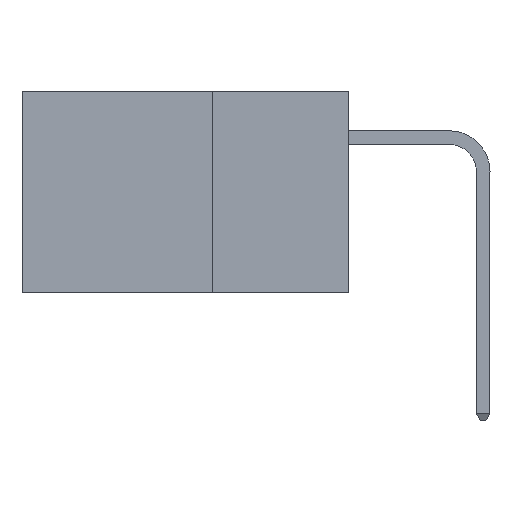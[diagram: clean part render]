
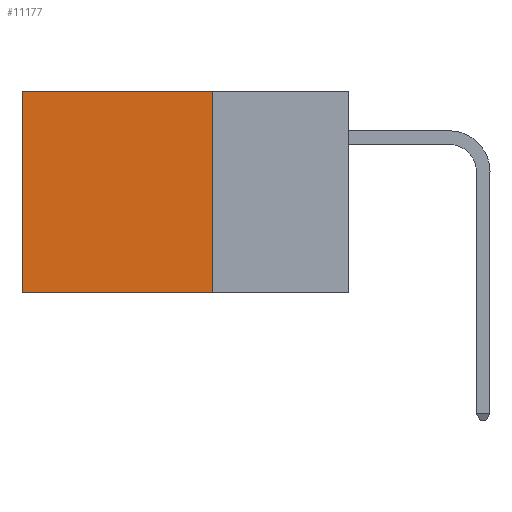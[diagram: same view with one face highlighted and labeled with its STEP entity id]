
A CAD part, left-side view. The second image highlights one B-rep face of the part: STEP entity #11177.
In plain terms, the highlighted planar face has unit normal (-1, 0, 0).
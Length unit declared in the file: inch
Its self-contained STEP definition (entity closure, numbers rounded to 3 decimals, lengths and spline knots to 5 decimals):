
#1679 = VECTOR ( 'NONE', #18552, 39.37008 ) ;
#2421 = EDGE_CURVE ( 'NONE', #29203, #9789, #13041, .T. ) ;
#3618 = CARTESIAN_POINT ( 'NONE',  ( 0.2875, 0.6, 0. ) ) ;
#3667 = EDGE_CURVE ( 'NONE', #9789, #4277, #11136, .T. ) ;
#3704 = CARTESIAN_POINT ( 'NONE',  ( 0.2875, 0.25, 0. ) ) ;
#4277 = VERTEX_POINT ( 'NONE', #32941 ) ;
#5396 = VECTOR ( 'NONE', #30680, 39.37008 ) ;
#6281 = DIRECTION ( 'NONE',  ( 0., 0., -1. ) ) ;
#8316 = LINE ( 'NONE', #9172, #29711 ) ;
#9172 = CARTESIAN_POINT ( 'NONE',  ( 0.2875, 0.25, 0. ) ) ;
#9330 = LINE ( 'NONE', #21212, #1679 ) ;
#9660 = VERTEX_POINT ( 'NONE', #18343 ) ;
#9789 = VERTEX_POINT ( 'NONE', #31069 ) ;
#11136 = LINE ( 'NONE', #3618, #25094 ) ;
#11177 = ADVANCED_FACE ( 'NONE', ( #20789 ), #28598, .F. ) ;
#11981 = CARTESIAN_POINT ( 'NONE',  ( 0.2875, 0.25, 0. ) ) ;
#13041 = LINE ( 'NONE', #26930, #5396 ) ;
#13064 = EDGE_LOOP ( 'NONE', ( #30244, #26776, #25489, #23297 ) ) ;
#13364 = EDGE_CURVE ( 'NONE', #29203, #9660, #8316, .T. ) ;
#14764 = DIRECTION ( 'NONE',  ( 0., 0., -1. ) ) ;
#14838 = DIRECTION ( 'NONE',  ( 0., 0., -1. ) ) ;
#18343 = CARTESIAN_POINT ( 'NONE',  ( 0.2875, 0.25, -0.37 ) ) ;
#18552 = DIRECTION ( 'NONE',  ( 0., 1., 0. ) ) ;
#20789 = FACE_OUTER_BOUND ( 'NONE', #13064, .T. ) ;
#21212 = CARTESIAN_POINT ( 'NONE',  ( 0.2875, 0.25, -0.37 ) ) ;
#23297 = ORIENTED_EDGE ( 'NONE', *, *, #2421, .T. ) ;
#25094 = VECTOR ( 'NONE', #14838, 39.37008 ) ;
#25489 = ORIENTED_EDGE ( 'NONE', *, *, #13364, .F. ) ;
#26776 = ORIENTED_EDGE ( 'NONE', *, *, #27947, .F. ) ;
#26930 = CARTESIAN_POINT ( 'NONE',  ( 0.2875, 0.25, 0. ) ) ;
#27947 = EDGE_CURVE ( 'NONE', #9660, #4277, #9330, .T. ) ;
#28598 = PLANE ( 'NONE',  #33181 ) ;
#29203 = VERTEX_POINT ( 'NONE', #3704 ) ;
#29711 = VECTOR ( 'NONE', #6281, 39.37008 ) ;
#30244 = ORIENTED_EDGE ( 'NONE', *, *, #3667, .T. ) ;
#30680 = DIRECTION ( 'NONE',  ( 0., 1., 0. ) ) ;
#31069 = CARTESIAN_POINT ( 'NONE',  ( 0.2875, 0.6, 0. ) ) ;
#31332 = DIRECTION ( 'NONE',  ( 1., 0., 0. ) ) ;
#32941 = CARTESIAN_POINT ( 'NONE',  ( 0.2875, 0.6, -0.37 ) ) ;
#33181 = AXIS2_PLACEMENT_3D ( 'NONE', #11981, #31332, #14764 ) ;
